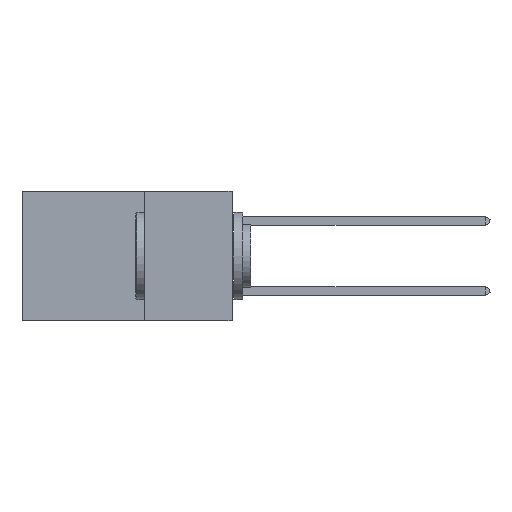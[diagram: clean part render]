
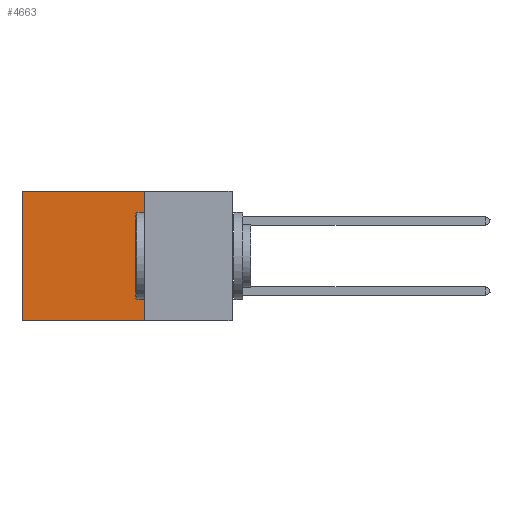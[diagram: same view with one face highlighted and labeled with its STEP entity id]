
A CAD part, left-side view. The second image highlights one B-rep face of the part: STEP entity #4663.
In plain terms, the highlighted planar face has unit normal (-1, 0, 0).
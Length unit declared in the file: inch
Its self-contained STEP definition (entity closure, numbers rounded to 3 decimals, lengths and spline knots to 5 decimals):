
#366 = DIRECTION ( 'NONE',  ( 1., 0., 0. ) ) ;
#451 = DIRECTION ( 'NONE',  ( 0., 0., -1. ) ) ;
#1261 = LINE ( 'NONE', #30492, #15995 ) ;
#1947 = VECTOR ( 'NONE', #451, 39.37008 ) ;
#3617 = CARTESIAN_POINT ( 'NONE',  ( 0.2875, 0.25, -0.37 ) ) ;
#3915 = DIRECTION ( 'NONE',  ( 0., 0., -1. ) ) ;
#4106 = CARTESIAN_POINT ( 'NONE',  ( 0.2875, 0.6, -0.37 ) ) ;
#4663 = ADVANCED_FACE ( 'NONE', ( #25287 ), #29544, .F. ) ;
#5633 = CARTESIAN_POINT ( 'NONE',  ( 0.2875, 0.25, 0. ) ) ;
#5848 = DIRECTION ( 'NONE',  ( 0., 0., -1. ) ) ;
#7734 = VECTOR ( 'NONE', #3915, 39.37008 ) ;
#7920 = ORIENTED_EDGE ( 'NONE', *, *, #29058, .T. ) ;
#9421 = EDGE_CURVE ( 'NONE', #29830, #30439, #24321, .T. ) ;
#10428 = VERTEX_POINT ( 'NONE', #15851 ) ;
#10858 = CARTESIAN_POINT ( 'NONE',  ( 0.2875, 0.6, 0. ) ) ;
#12118 = ORIENTED_EDGE ( 'NONE', *, *, #20402, .T. ) ;
#14203 = CARTESIAN_POINT ( 'NONE',  ( 0.2875, 0.25, 0. ) ) ;
#14814 = VECTOR ( 'NONE', #27232, 39.37008 ) ;
#15851 = CARTESIAN_POINT ( 'NONE',  ( 0.2875, 0.6, 0. ) ) ;
#15995 = VECTOR ( 'NONE', #17654, 39.37008 ) ;
#16257 = ORIENTED_EDGE ( 'NONE', *, *, #31094, .F. ) ;
#16600 = CARTESIAN_POINT ( 'NONE',  ( 0.2875, 0.25, -0.37 ) ) ;
#16973 = CARTESIAN_POINT ( 'NONE',  ( 0.2875, 0.25, 0. ) ) ;
#17654 = DIRECTION ( 'NONE',  ( 0., 1., 0. ) ) ;
#19236 = ORIENTED_EDGE ( 'NONE', *, *, #9421, .F. ) ;
#20402 = EDGE_CURVE ( 'NONE', #31609, #10428, #1261, .T. ) ;
#20649 = AXIS2_PLACEMENT_3D ( 'NONE', #5633, #366, #5848 ) ;
#21193 = LINE ( 'NONE', #10858, #1947 ) ;
#24321 = LINE ( 'NONE', #16600, #14814 ) ;
#24969 = EDGE_LOOP ( 'NONE', ( #7920, #19236, #16257, #12118 ) ) ;
#25287 = FACE_OUTER_BOUND ( 'NONE', #24969, .T. ) ;
#27232 = DIRECTION ( 'NONE',  ( 0., 1., 0. ) ) ;
#29058 = EDGE_CURVE ( 'NONE', #10428, #30439, #21193, .T. ) ;
#29544 = PLANE ( 'NONE',  #20649 ) ;
#29830 = VERTEX_POINT ( 'NONE', #3617 ) ;
#30439 = VERTEX_POINT ( 'NONE', #4106 ) ;
#30492 = CARTESIAN_POINT ( 'NONE',  ( 0.2875, 0.25, 0. ) ) ;
#31094 = EDGE_CURVE ( 'NONE', #31609, #29830, #33697, .T. ) ;
#31609 = VERTEX_POINT ( 'NONE', #16973 ) ;
#33697 = LINE ( 'NONE', #14203, #7734 ) ;
